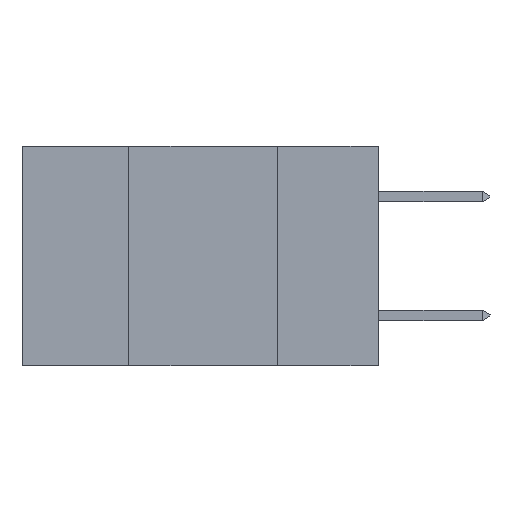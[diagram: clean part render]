
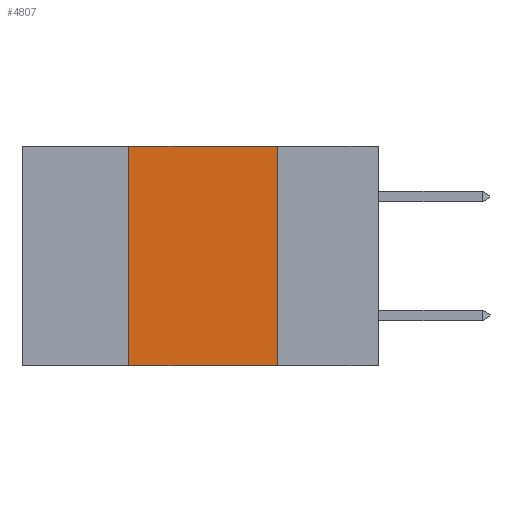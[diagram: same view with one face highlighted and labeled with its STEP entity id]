
A CAD part, left-side view. The second image highlights one B-rep face of the part: STEP entity #4807.
In plain terms, the highlighted planar face has unit normal (-1, 0, 0).
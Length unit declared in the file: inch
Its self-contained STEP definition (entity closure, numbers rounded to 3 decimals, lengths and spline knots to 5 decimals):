
#470 = DIRECTION ( 'NONE',  ( 0., 0., -1. ) ) ;
#2383 = CARTESIAN_POINT ( 'NONE',  ( 0., 0.6, -0.37 ) ) ;
#2576 = VECTOR ( 'NONE', #17137, 39.37008 ) ;
#3132 = ORIENTED_EDGE ( 'NONE', *, *, #13584, .T. ) ;
#3885 = VECTOR ( 'NONE', #12737, 39.37008 ) ;
#4296 = EDGE_CURVE ( 'NONE', #8228, #25744, #10461, .T. ) ;
#4480 = EDGE_CURVE ( 'NONE', #4827, #12769, #18770, .T. ) ;
#4585 = VECTOR ( 'NONE', #12269, 39.37008 ) ;
#4775 = CARTESIAN_POINT ( 'NONE',  ( 0., 0.42, 0. ) ) ;
#4807 = ADVANCED_FACE ( 'NONE', ( #7264 ), #24979, .F. ) ;
#4827 = VERTEX_POINT ( 'NONE', #4858 ) ;
#4858 = CARTESIAN_POINT ( 'NONE',  ( 0., 0.42, -0.37 ) ) ;
#5469 = LINE ( 'NONE', #2383, #3885 ) ;
#6641 = CARTESIAN_POINT ( 'NONE',  ( 0., 0.17, -0.37 ) ) ;
#7264 = FACE_OUTER_BOUND ( 'NONE', #23504, .T. ) ;
#8228 = VERTEX_POINT ( 'NONE', #18827 ) ;
#8705 = AXIS2_PLACEMENT_3D ( 'NONE', #19145, #23181, #11021 ) ;
#10461 = LINE ( 'NONE', #16690, #13943 ) ;
#11021 = DIRECTION ( 'NONE',  ( 0., 0., -1. ) ) ;
#12192 = ORIENTED_EDGE ( 'NONE', *, *, #19080, .F. ) ;
#12269 = DIRECTION ( 'NONE',  ( 0., -1., 0. ) ) ;
#12737 = DIRECTION ( 'NONE',  ( 0., -1., 0. ) ) ;
#12769 = VERTEX_POINT ( 'NONE', #4775 ) ;
#13543 = CARTESIAN_POINT ( 'NONE',  ( 0., 0.6, 0. ) ) ;
#13584 = EDGE_CURVE ( 'NONE', #4827, #25744, #5469, .T. ) ;
#13943 = VECTOR ( 'NONE', #470, 39.37008 ) ;
#15548 = ORIENTED_EDGE ( 'NONE', *, *, #4296, .F. ) ;
#16303 = ORIENTED_EDGE ( 'NONE', *, *, #4480, .F. ) ;
#16690 = CARTESIAN_POINT ( 'NONE',  ( 0., 0.17, 0. ) ) ;
#17137 = DIRECTION ( 'NONE',  ( 0., 0., 1. ) ) ;
#18770 = LINE ( 'NONE', #22835, #2576 ) ;
#18827 = CARTESIAN_POINT ( 'NONE',  ( 0., 0.17, 0. ) ) ;
#19080 = EDGE_CURVE ( 'NONE', #12769, #8228, #26148, .T. ) ;
#19145 = CARTESIAN_POINT ( 'NONE',  ( 0., 0.6, 0. ) ) ;
#22835 = CARTESIAN_POINT ( 'NONE',  ( 0., 0.42, 0. ) ) ;
#23181 = DIRECTION ( 'NONE',  ( 1., 0., 0. ) ) ;
#23504 = EDGE_LOOP ( 'NONE', ( #15548, #12192, #16303, #3132 ) ) ;
#24979 = PLANE ( 'NONE',  #8705 ) ;
#25744 = VERTEX_POINT ( 'NONE', #6641 ) ;
#26148 = LINE ( 'NONE', #13543, #4585 ) ;
